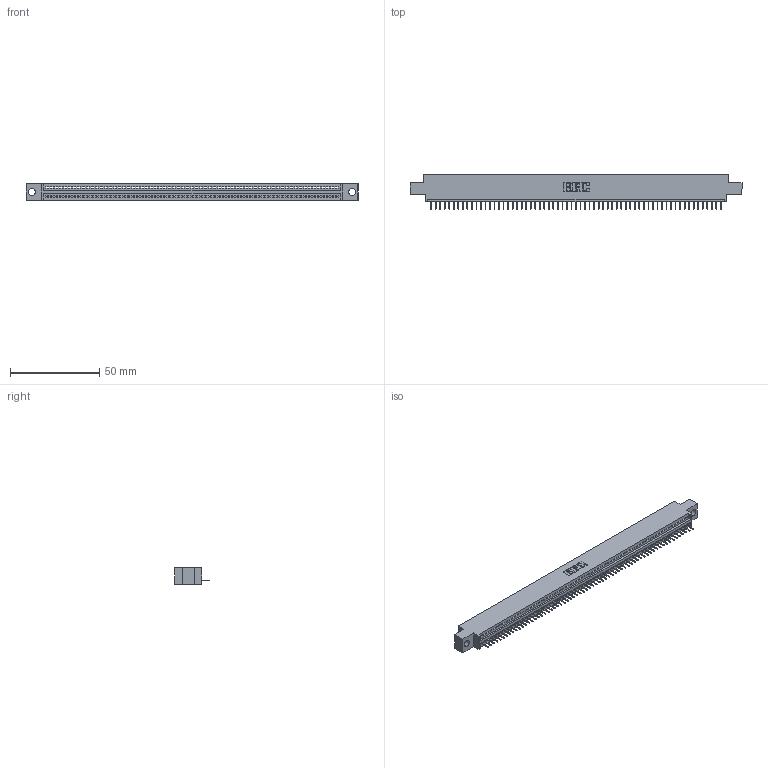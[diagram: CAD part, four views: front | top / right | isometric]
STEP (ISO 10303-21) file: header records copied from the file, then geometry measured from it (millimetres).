
FILE_DESCRIPTION (( 'STEP AP203' ), '1' );
FILE_NAME ('395-065-524-604.STEP', '2021-05-31T22:02:58', ( '' ), ( '' ), 'SwSTEP 2.0', 'SolidWorks 2020', '' );
FILE_SCHEMA (( 'CONFIG_CONTROL_DESIGN' ));
Length unit declared in the file: inch
Products named in the file (3): 345 Part_0.170 Offset - 0.156 Dia-TI; 345-292-001_345-293-124; 395-065-524-604
Assembly tree (66 placements, depth 2):
  395-065-524-604
    345 Part_0.170 Offset - 0.156 Dia-TI
    345-292-001_345-293-124  x65
Bounding box: 186.31 x 19.35 x 9.4 mm (x, y, z)
Volume: 17408.1 mm3; surface area: 22594.5 mm2
Topology: 66 solids, 66 shells, 4174 faces, 12089 edges, 7798 vertices
Faces by surface type: plane 3088, cylinder 1086
Entity records: 46449 total; most frequent: CARTESIAN_POINT 8053, ORIENTED_EDGE 8050, DIRECTION 6999, EDGE_CURVE 4025, VECTOR 3637, LINE 3637, VERTEX_POINT 2678, AXIS2_PLACEMENT_3D 1681
